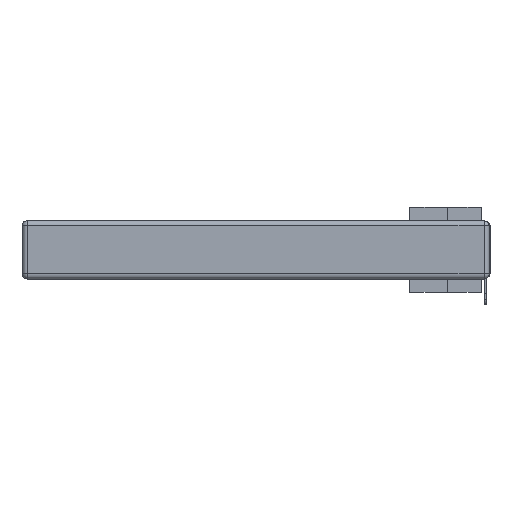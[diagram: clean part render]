
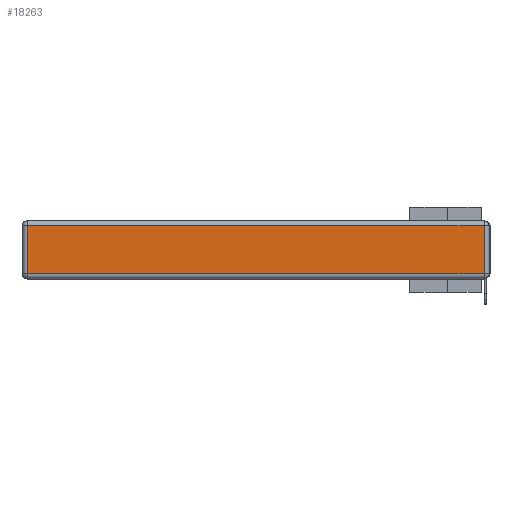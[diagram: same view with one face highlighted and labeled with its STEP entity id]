
A CAD part, left-side view. The second image highlights one B-rep face of the part: STEP entity #18263.
In plain terms, the highlighted planar face has unit normal (-1, 0, 0).
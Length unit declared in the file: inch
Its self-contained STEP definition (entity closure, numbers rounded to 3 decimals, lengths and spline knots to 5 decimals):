
#1171 = EDGE_LOOP ( 'NONE', ( #24107, #15771, #7568, #28566 ) ) ;
#1570 = CARTESIAN_POINT ( 'NONE',  ( 0., 0., -0.313 ) ) ;
#1581 = DIRECTION ( 'NONE',  ( -1., 0., 0. ) ) ;
#5902 = CARTESIAN_POINT ( 'NONE',  ( 0., 2.75, -0.03 ) ) ;
#7568 = ORIENTED_EDGE ( 'NONE', *, *, #21442, .T. ) ;
#8003 = VECTOR ( 'NONE', #15434, 39.37008 ) ;
#8795 = CARTESIAN_POINT ( 'NONE',  ( 0., 2.72, -0.03 ) ) ;
#9177 = EDGE_CURVE ( 'NONE', #16795, #11693, #23032, .T. ) ;
#9933 = EDGE_CURVE ( 'NONE', #24111, #16795, #24981, .T. ) ;
#10611 = DIRECTION ( 'NONE',  ( 0., 0., 1. ) ) ;
#10909 = CARTESIAN_POINT ( 'NONE',  ( 0., 2.72, -0.313 ) ) ;
#11448 = DIRECTION ( 'NONE',  ( 0., -1., 0. ) ) ;
#11693 = VERTEX_POINT ( 'NONE', #20101 ) ;
#11753 = AXIS2_PLACEMENT_3D ( 'NONE', #23043, #1581, #21022 ) ;
#11982 = VECTOR ( 'NONE', #11448, 39.37008 ) ;
#12951 = LINE ( 'NONE', #5902, #24872 ) ;
#15434 = DIRECTION ( 'NONE',  ( 0., 0., -1. ) ) ;
#15454 = DIRECTION ( 'NONE',  ( 0., 1., 0. ) ) ;
#15771 = ORIENTED_EDGE ( 'NONE', *, *, #25834, .T. ) ;
#16795 = VERTEX_POINT ( 'NONE', #10909 ) ;
#18263 = ADVANCED_FACE ( 'NONE', ( #30220 ), #23192, .T. ) ;
#20101 = CARTESIAN_POINT ( 'NONE',  ( 0., 0.03, -0.313 ) ) ;
#20744 = VERTEX_POINT ( 'NONE', #30916 ) ;
#21022 = DIRECTION ( 'NONE',  ( 0., 0., 1. ) ) ;
#21442 = EDGE_CURVE ( 'NONE', #20744, #24111, #12951, .T. ) ;
#22653 = LINE ( 'NONE', #29837, #23029 ) ;
#23029 = VECTOR ( 'NONE', #10611, 39.37008 ) ;
#23032 = LINE ( 'NONE', #1570, #11982 ) ;
#23043 = CARTESIAN_POINT ( 'NONE',  ( 0., 0., -0.343 ) ) ;
#23192 = PLANE ( 'NONE',  #11753 ) ;
#24107 = ORIENTED_EDGE ( 'NONE', *, *, #9177, .T. ) ;
#24111 = VERTEX_POINT ( 'NONE', #8795 ) ;
#24872 = VECTOR ( 'NONE', #15454, 39.37008 ) ;
#24981 = LINE ( 'NONE', #27320, #8003 ) ;
#25834 = EDGE_CURVE ( 'NONE', #11693, #20744, #22653, .T. ) ;
#27320 = CARTESIAN_POINT ( 'NONE',  ( 0., 2.72, -0.343 ) ) ;
#28566 = ORIENTED_EDGE ( 'NONE', *, *, #9933, .T. ) ;
#29837 = CARTESIAN_POINT ( 'NONE',  ( 0., 0.03, -0.343 ) ) ;
#30220 = FACE_OUTER_BOUND ( 'NONE', #1171, .T. ) ;
#30916 = CARTESIAN_POINT ( 'NONE',  ( 0., 0.03, -0.03 ) ) ;
